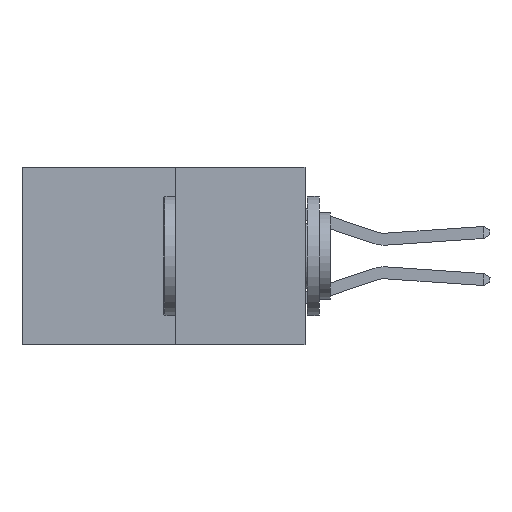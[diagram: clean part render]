
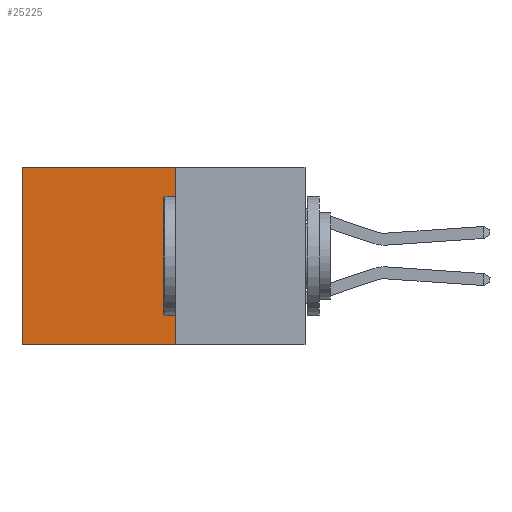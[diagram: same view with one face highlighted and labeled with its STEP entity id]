
A CAD part, left-side view. The second image highlights one B-rep face of the part: STEP entity #25225.
In plain terms, the highlighted planar face has unit normal (-1, 0, 0).
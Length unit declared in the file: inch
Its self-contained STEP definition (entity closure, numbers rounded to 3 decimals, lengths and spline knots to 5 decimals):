
#21 = CARTESIAN_POINT ( 'NONE',  ( 0.277, 0.27, -0.37 ) ) ;
#99 = EDGE_CURVE ( 'NONE', #24007, #20876, #6429, .T. ) ;
#937 = DIRECTION ( 'NONE',  ( 0., 0., -1. ) ) ;
#971 = VECTOR ( 'NONE', #17918, 39.37008 ) ;
#1392 = CARTESIAN_POINT ( 'NONE',  ( 0.277, 0.27, 0. ) ) ;
#2997 = ORIENTED_EDGE ( 'NONE', *, *, #99, .T. ) ;
#3009 = CARTESIAN_POINT ( 'NONE',  ( 0.277, 0.27, -0.37 ) ) ;
#4303 = CARTESIAN_POINT ( 'NONE',  ( 0.277, 0.59, -0.37 ) ) ;
#4849 = EDGE_LOOP ( 'NONE', ( #2997, #29322, #10622, #7594 ) ) ;
#5855 = EDGE_CURVE ( 'NONE', #25398, #9012, #21919, .T. ) ;
#6429 = LINE ( 'NONE', #18750, #971 ) ;
#7347 = VECTOR ( 'NONE', #24399, 39.37008 ) ;
#7594 = ORIENTED_EDGE ( 'NONE', *, *, #15232, .T. ) ;
#9012 = VERTEX_POINT ( 'NONE', #3009 ) ;
#9037 = VECTOR ( 'NONE', #937, 39.37008 ) ;
#10622 = ORIENTED_EDGE ( 'NONE', *, *, #5855, .F. ) ;
#12027 = CARTESIAN_POINT ( 'NONE',  ( 0.277, 0.59, 0. ) ) ;
#12468 = CARTESIAN_POINT ( 'NONE',  ( 0.277, 0.27, -0.37 ) ) ;
#12612 = CARTESIAN_POINT ( 'NONE',  ( 0.277, 0.27, -0.37 ) ) ;
#13289 = VECTOR ( 'NONE', #19171, 39.37008 ) ;
#14899 = DIRECTION ( 'NONE',  ( 0., 0., -1. ) ) ;
#15232 = EDGE_CURVE ( 'NONE', #25398, #24007, #24858, .T. ) ;
#17686 = CARTESIAN_POINT ( 'NONE',  ( 0.277, 0.27, 0. ) ) ;
#17918 = DIRECTION ( 'NONE',  ( 0., 0., -1. ) ) ;
#18750 = CARTESIAN_POINT ( 'NONE',  ( 0.277, 0.59, -0.37 ) ) ;
#19171 = DIRECTION ( 'NONE',  ( 0., 1., 0. ) ) ;
#19987 = FACE_OUTER_BOUND ( 'NONE', #4849, .T. ) ;
#20876 = VERTEX_POINT ( 'NONE', #4303 ) ;
#21919 = LINE ( 'NONE', #21, #9037 ) ;
#23441 = EDGE_CURVE ( 'NONE', #9012, #20876, #25404, .T. ) ;
#23968 = PLANE ( 'NONE',  #28273 ) ;
#24007 = VERTEX_POINT ( 'NONE', #12027 ) ;
#24399 = DIRECTION ( 'NONE',  ( 0., 1., 0. ) ) ;
#24858 = LINE ( 'NONE', #1392, #7347 ) ;
#25225 = ADVANCED_FACE ( 'NONE', ( #19987 ), #23968, .F. ) ;
#25398 = VERTEX_POINT ( 'NONE', #17686 ) ;
#25404 = LINE ( 'NONE', #12468, #13289 ) ;
#28273 = AXIS2_PLACEMENT_3D ( 'NONE', #12612, #28552, #14899 ) ;
#28552 = DIRECTION ( 'NONE',  ( 1., 0., 0. ) ) ;
#29322 = ORIENTED_EDGE ( 'NONE', *, *, #23441, .F. ) ;
